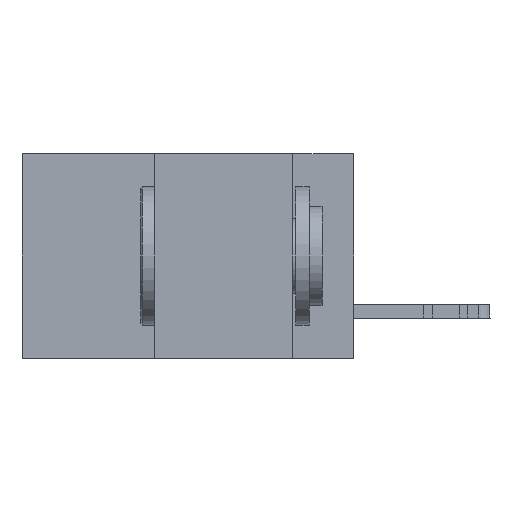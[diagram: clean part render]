
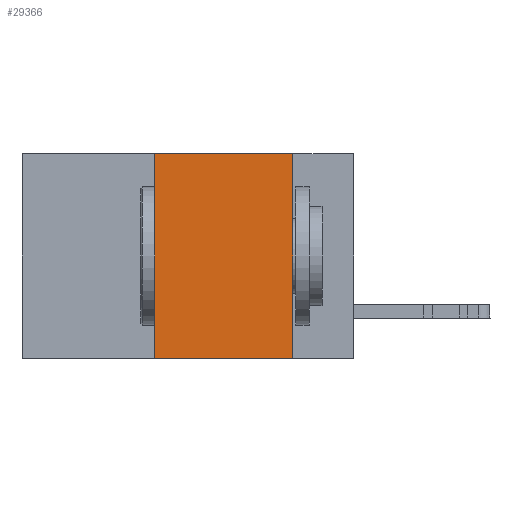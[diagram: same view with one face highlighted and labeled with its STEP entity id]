
A CAD part, left-side view. The second image highlights one B-rep face of the part: STEP entity #29366.
In plain terms, the highlighted planar face has unit normal (-1, 0, 0).
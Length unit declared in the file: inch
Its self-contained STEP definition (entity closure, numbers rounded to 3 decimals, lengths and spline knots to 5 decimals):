
#288 = VECTOR ( 'NONE', #18326, 39.37008 ) ;
#629 = VERTEX_POINT ( 'NONE', #25025 ) ;
#2191 = PLANE ( 'NONE',  #15162 ) ;
#2416 = LINE ( 'NONE', #14881, #21229 ) ;
#3359 = CARTESIAN_POINT ( 'NONE',  ( 0., 0.6, 0. ) ) ;
#3496 = ORIENTED_EDGE ( 'NONE', *, *, #11215, .F. ) ;
#4180 = VERTEX_POINT ( 'NONE', #30577 ) ;
#8521 = DIRECTION ( 'NONE',  ( 0., 0., -1. ) ) ;
#8874 = VECTOR ( 'NONE', #12957, 39.37008 ) ;
#9890 = LINE ( 'NONE', #3359, #8874 ) ;
#10873 = ORIENTED_EDGE ( 'NONE', *, *, #33224, .F. ) ;
#11215 = EDGE_CURVE ( 'NONE', #629, #4180, #25048, .T. ) ;
#12957 = DIRECTION ( 'NONE',  ( 0., -1., 0. ) ) ;
#13334 = VECTOR ( 'NONE', #21354, 39.37008 ) ;
#14654 = CARTESIAN_POINT ( 'NONE',  ( 0., 0.6, 0. ) ) ;
#14817 = CARTESIAN_POINT ( 'NONE',  ( 0., 0.6, -0.37 ) ) ;
#14881 = CARTESIAN_POINT ( 'NONE',  ( 0., 0.36, 0. ) ) ;
#15162 = AXIS2_PLACEMENT_3D ( 'NONE', #14654, #27107, #8521 ) ;
#15275 = DIRECTION ( 'NONE',  ( 0., 0., 1. ) ) ;
#15350 = CARTESIAN_POINT ( 'NONE',  ( 0., 0.36, -0.37 ) ) ;
#15898 = ORIENTED_EDGE ( 'NONE', *, *, #39424, .F. ) ;
#18326 = DIRECTION ( 'NONE',  ( 0., 0., -1. ) ) ;
#21229 = VECTOR ( 'NONE', #15275, 39.37008 ) ;
#21354 = DIRECTION ( 'NONE',  ( 0., -1., 0. ) ) ;
#22398 = VERTEX_POINT ( 'NONE', #28922 ) ;
#25025 = CARTESIAN_POINT ( 'NONE',  ( 0., 0.11, 0. ) ) ;
#25048 = LINE ( 'NONE', #31366, #288 ) ;
#26043 = EDGE_LOOP ( 'NONE', ( #3496, #10873, #15898, #31491 ) ) ;
#27107 = DIRECTION ( 'NONE',  ( 1., 0., 0. ) ) ;
#27817 = VERTEX_POINT ( 'NONE', #15350 ) ;
#28922 = CARTESIAN_POINT ( 'NONE',  ( 0., 0.36, 0. ) ) ;
#29366 = ADVANCED_FACE ( 'NONE', ( #33446 ), #2191, .F. ) ;
#30577 = CARTESIAN_POINT ( 'NONE',  ( 0., 0.11, -0.37 ) ) ;
#31125 = LINE ( 'NONE', #14817, #13334 ) ;
#31366 = CARTESIAN_POINT ( 'NONE',  ( 0., 0.11, 0. ) ) ;
#31491 = ORIENTED_EDGE ( 'NONE', *, *, #36927, .T. ) ;
#33224 = EDGE_CURVE ( 'NONE', #22398, #629, #9890, .T. ) ;
#33446 = FACE_OUTER_BOUND ( 'NONE', #26043, .T. ) ;
#36927 = EDGE_CURVE ( 'NONE', #27817, #4180, #31125, .T. ) ;
#39424 = EDGE_CURVE ( 'NONE', #27817, #22398, #2416, .T. ) ;
